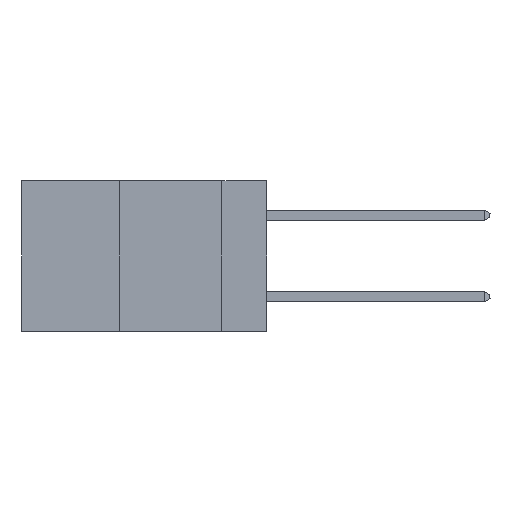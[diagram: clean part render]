
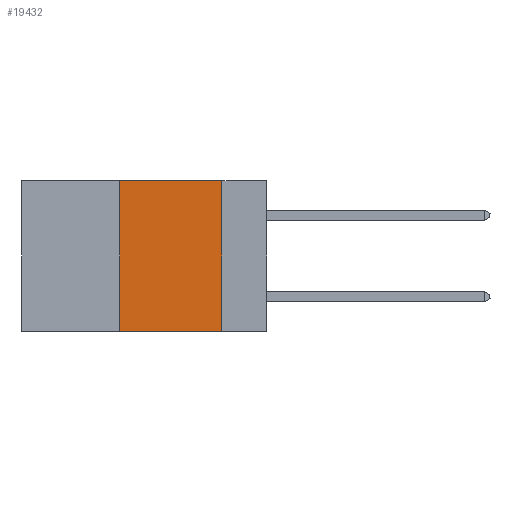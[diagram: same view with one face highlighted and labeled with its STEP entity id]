
A CAD part, left-side view. The second image highlights one B-rep face of the part: STEP entity #19432.
In plain terms, the highlighted planar face has unit normal (-1, 0, 0).
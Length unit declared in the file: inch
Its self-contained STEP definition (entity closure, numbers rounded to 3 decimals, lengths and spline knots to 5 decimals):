
#1547 = CARTESIAN_POINT ( 'NONE',  ( 0., 0.11, 0. ) ) ;
#2081 = CARTESIAN_POINT ( 'NONE',  ( 0., 0.6, 0. ) ) ;
#2603 = CARTESIAN_POINT ( 'NONE',  ( 0., 0.11, -0.37 ) ) ;
#3043 = VECTOR ( 'NONE', #5594, 39.37008 ) ;
#4209 = CARTESIAN_POINT ( 'NONE',  ( 0., 0.11, 0. ) ) ;
#4289 = DIRECTION ( 'NONE',  ( 0., 0., -1. ) ) ;
#5151 = DIRECTION ( 'NONE',  ( 0., -1., 0. ) ) ;
#5174 = EDGE_CURVE ( 'NONE', #8164, #22943, #8317, .T. ) ;
#5231 = VERTEX_POINT ( 'NONE', #1547 ) ;
#5594 = DIRECTION ( 'NONE',  ( 0., 0., 1. ) ) ;
#6353 = DIRECTION ( 'NONE',  ( 0., 0., -1. ) ) ;
#6415 = VECTOR ( 'NONE', #5151, 39.37008 ) ;
#6607 = ORIENTED_EDGE ( 'NONE', *, *, #5174, .T. ) ;
#6617 = ORIENTED_EDGE ( 'NONE', *, *, #23427, .F. ) ;
#7366 = ORIENTED_EDGE ( 'NONE', *, *, #17909, .F. ) ;
#8164 = VERTEX_POINT ( 'NONE', #14329 ) ;
#8317 = LINE ( 'NONE', #18351, #24968 ) ;
#9817 = CARTESIAN_POINT ( 'NONE',  ( 0., 0.36, 0. ) ) ;
#10642 = PLANE ( 'NONE',  #20571 ) ;
#11234 = EDGE_LOOP ( 'NONE', ( #6617, #20066, #7366, #6607 ) ) ;
#12285 = LINE ( 'NONE', #4209, #22700 ) ;
#14163 = CARTESIAN_POINT ( 'NONE',  ( 0., 0.36, 0. ) ) ;
#14329 = CARTESIAN_POINT ( 'NONE',  ( 0., 0.36, -0.37 ) ) ;
#15029 = LINE ( 'NONE', #9817, #3043 ) ;
#15461 = VERTEX_POINT ( 'NONE', #14163 ) ;
#15921 = FACE_OUTER_BOUND ( 'NONE', #11234, .T. ) ;
#16971 = DIRECTION ( 'NONE',  ( 1., 0., 0. ) ) ;
#17653 = LINE ( 'NONE', #19863, #6415 ) ;
#17781 = EDGE_CURVE ( 'NONE', #15461, #5231, #17653, .T. ) ;
#17909 = EDGE_CURVE ( 'NONE', #8164, #15461, #15029, .T. ) ;
#18351 = CARTESIAN_POINT ( 'NONE',  ( 0., 0.6, -0.37 ) ) ;
#19432 = ADVANCED_FACE ( 'NONE', ( #15921 ), #10642, .F. ) ;
#19863 = CARTESIAN_POINT ( 'NONE',  ( 0., 0.6, 0. ) ) ;
#20066 = ORIENTED_EDGE ( 'NONE', *, *, #17781, .F. ) ;
#20571 = AXIS2_PLACEMENT_3D ( 'NONE', #2081, #16971, #4289 ) ;
#22700 = VECTOR ( 'NONE', #6353, 39.37008 ) ;
#22943 = VERTEX_POINT ( 'NONE', #2603 ) ;
#23427 = EDGE_CURVE ( 'NONE', #5231, #22943, #12285, .T. ) ;
#24968 = VECTOR ( 'NONE', #26570, 39.37008 ) ;
#26570 = DIRECTION ( 'NONE',  ( 0., -1., 0. ) ) ;
